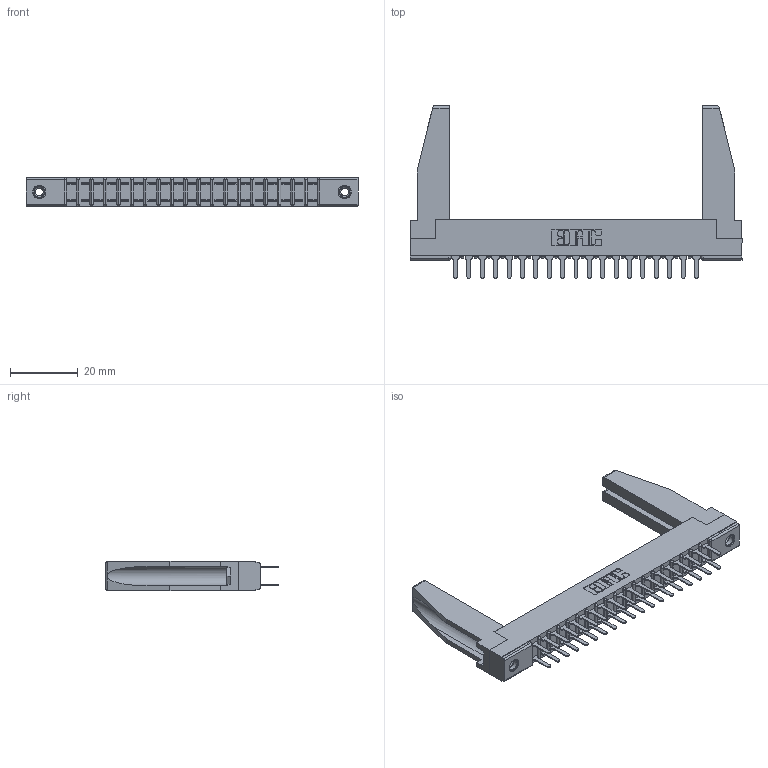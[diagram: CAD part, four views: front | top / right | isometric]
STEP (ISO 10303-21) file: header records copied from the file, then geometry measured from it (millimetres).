
FILE_DESCRIPTION (( 'STEP AP203' ), '1' );
FILE_NAME ('357-038-520-278.STEP', '2019-09-18T04:04:49', ( '' ), ( '' ), 'SwSTEP 2.0', 'SolidWorks 2016', '' );
FILE_SCHEMA (( 'CONFIG_CONTROL_DESIGN' ));
Length unit declared in the file: inch
Products named in the file (5): 357-038-520-278; 307 Part_.156 Dia Mounting Holes; 345-250-001_345-250-001-102; 307-290-001_520; 307-220-078
Assembly tree (43 placements, depth 2):
  357-038-520-278
    307 Part_.156 Dia Mounting Holes
    307-290-001_520  x38
    307-220-078  x2
    345-250-001_345-250-001-102  x2
Bounding box: 98.3 x 51.13 x 8.71 mm (x, y, z)
Volume: 10451.3 mm3; surface area: 15178.2 mm2
Topology: 43 solids, 43 shells, 2016 faces, 5593 edges, 3614 vertices
Faces by surface type: plane 1332, cylinder 628, sphere 40, cone 12, torus 4
Entity records: 22139 total; most frequent: CARTESIAN_POINT 3637, ORIENTED_EDGE 3560, DIRECTION 3526, EDGE_CURVE 1780, LINE 1360, VECTOR 1360, VERTEX_POINT 1152, AXIS2_PLACEMENT_3D 1083
